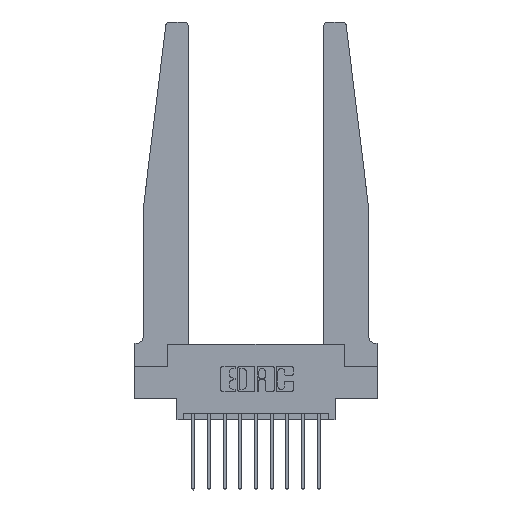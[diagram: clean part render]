
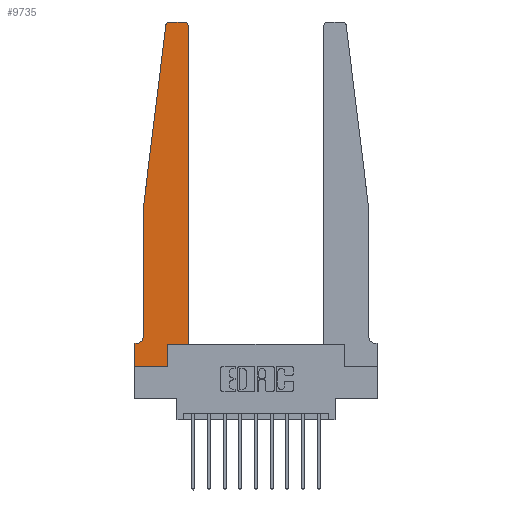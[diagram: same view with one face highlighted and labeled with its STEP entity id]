
A CAD part, top view. The second image highlights one B-rep face of the part: STEP entity #9735.
In plain terms, the highlighted planar face has unit normal (0, 0, 1).
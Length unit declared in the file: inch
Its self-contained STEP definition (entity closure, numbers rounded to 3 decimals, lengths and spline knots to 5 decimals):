
#24 = CARTESIAN_POINT ( 'NONE',  ( 0.27653, 2.72, 0.37 ) ) ;
#117 = VECTOR ( 'NONE', #2844, 39.37008 ) ;
#238 = VERTEX_POINT ( 'NONE', #4999 ) ;
#250 = VERTEX_POINT ( 'NONE', #1416 ) ;
#316 = LINE ( 'NONE', #969, #6239 ) ;
#325 = DIRECTION ( 'NONE',  ( -1., 0., 0. ) ) ;
#347 = LINE ( 'NONE', #9294, #12099 ) ;
#415 = ORIENTED_EDGE ( 'NONE', *, *, #4697, .T. ) ;
#616 = EDGE_CURVE ( 'NONE', #13583, #8417, #14732, .T. ) ;
#830 = CARTESIAN_POINT ( 'NONE',  ( 0.395, 2.72, 0.37 ) ) ;
#891 = ORIENTED_EDGE ( 'NONE', *, *, #8493, .T. ) ;
#969 = CARTESIAN_POINT ( 'NONE',  ( 0.065, 1.25, 0.37 ) ) ;
#978 = EDGE_CURVE ( 'NONE', #8793, #11967, #13027, .T. ) ;
#1045 = CARTESIAN_POINT ( 'NONE',  ( 0.2605, 0.18, 0.37 ) ) ;
#1146 = EDGE_CURVE ( 'NONE', #4837, #238, #4640, .T. ) ;
#1221 = DIRECTION ( 'NONE',  ( 1., 0., 0. ) ) ;
#1333 = ORIENTED_EDGE ( 'NONE', *, *, #1146, .T. ) ;
#1416 = CARTESIAN_POINT ( 'NONE',  ( 0.015, 0.1875, 0.37 ) ) ;
#1560 = EDGE_LOOP ( 'NONE', ( #9236, #891, #6658, #9696, #10769, #415, #2440, #8601, #11842, #1333, #6255, #4592 ) ) ;
#1651 = CARTESIAN_POINT ( 'NONE',  ( 0.065, 1.25, 0.37 ) ) ;
#1719 = CARTESIAN_POINT ( 'NONE',  ( 0.2605, 0.18, 0.37 ) ) ;
#1754 = CARTESIAN_POINT ( 'NONE',  ( 0.425, 0.18, 0.37 ) ) ;
#1831 = EDGE_CURVE ( 'NONE', #12638, #8793, #347, .T. ) ;
#2023 = DIRECTION ( 'NONE',  ( 1., 0., 0. ) ) ;
#2075 = FACE_OUTER_BOUND ( 'NONE', #1560, .T. ) ;
#2248 = DIRECTION ( 'NONE',  ( 0., 1., 0. ) ) ;
#2430 = EDGE_CURVE ( 'NONE', #8417, #10981, #4631, .T. ) ;
#2440 = ORIENTED_EDGE ( 'NONE', *, *, #1831, .T. ) ;
#2844 = DIRECTION ( 'NONE',  ( 0., -1., 0. ) ) ;
#3361 = DIRECTION ( 'NONE',  ( -0.122, -0.992, 0. ) ) ;
#3712 = AXIS2_PLACEMENT_3D ( 'NONE', #14414, #7411, #325 ) ;
#4321 = AXIS2_PLACEMENT_3D ( 'NONE', #830, #9087, #2023 ) ;
#4592 = ORIENTED_EDGE ( 'NONE', *, *, #616, .T. ) ;
#4631 = LINE ( 'NONE', #5752, #10487 ) ;
#4640 = LINE ( 'NONE', #1754, #10501 ) ;
#4697 = EDGE_CURVE ( 'NONE', #250, #12638, #8228, .T. ) ;
#4837 = VERTEX_POINT ( 'NONE', #1719 ) ;
#4999 = CARTESIAN_POINT ( 'NONE',  ( 0.425, 0.18, 0.37 ) ) ;
#5190 = DIRECTION ( 'NONE',  ( 0., 0., 1. ) ) ;
#5752 = CARTESIAN_POINT ( 'NONE',  ( 0.25, 2.75, 0.37 ) ) ;
#6239 = VECTOR ( 'NONE', #3361, 39.37008 ) ;
#6249 = CARTESIAN_POINT ( 'NONE',  ( 0., 0., 0.37 ) ) ;
#6255 = ORIENTED_EDGE ( 'NONE', *, *, #8692, .T. ) ;
#6658 = ORIENTED_EDGE ( 'NONE', *, *, #12564, .T. ) ;
#7308 = CARTESIAN_POINT ( 'NONE',  ( 0.24675, 2.72367, 0.37 ) ) ;
#7411 = DIRECTION ( 'NONE',  ( 0., 0., -1. ) ) ;
#7706 = CARTESIAN_POINT ( 'NONE',  ( 0.425, 2.72, 0.37 ) ) ;
#7771 = CARTESIAN_POINT ( 'NONE',  ( 0.065, 1.25, 0.37 ) ) ;
#8195 = CARTESIAN_POINT ( 'NONE',  ( 0., 0.1875, 0.37 ) ) ;
#8228 = LINE ( 'NONE', #13088, #10969 ) ;
#8288 = DIRECTION ( 'NONE',  ( 0., 0., 1. ) ) ;
#8417 = VERTEX_POINT ( 'NONE', #12748 ) ;
#8493 = EDGE_CURVE ( 'NONE', #10981, #13328, #11287, .T. ) ;
#8601 = ORIENTED_EDGE ( 'NONE', *, *, #978, .T. ) ;
#8645 = CARTESIAN_POINT ( 'NONE',  ( 0.425, 0.18, 0.37 ) ) ;
#8692 = EDGE_CURVE ( 'NONE', #238, #13583, #14959, .T. ) ;
#8731 = CIRCLE ( 'NONE', #3712, 0.05 ) ;
#8793 = VERTEX_POINT ( 'NONE', #14630 ) ;
#9006 = VECTOR ( 'NONE', #2248, 39.37008 ) ;
#9087 = DIRECTION ( 'NONE',  ( 0., 0., 1. ) ) ;
#9177 = EDGE_CURVE ( 'NONE', #10289, #250, #8731, .T. ) ;
#9236 = ORIENTED_EDGE ( 'NONE', *, *, #2430, .T. ) ;
#9294 = CARTESIAN_POINT ( 'NONE',  ( 0., 0., 0.37 ) ) ;
#9696 = ORIENTED_EDGE ( 'NONE', *, *, #12857, .T. ) ;
#9735 = ADVANCED_FACE ( 'NONE', ( #2075 ), #12166, .T. ) ;
#9979 = VECTOR ( 'NONE', #10912, 39.37008 ) ;
#10289 = VERTEX_POINT ( 'NONE', #14479 ) ;
#10487 = VECTOR ( 'NONE', #15109, 39.37008 ) ;
#10501 = VECTOR ( 'NONE', #14646, 39.37008 ) ;
#10769 = ORIENTED_EDGE ( 'NONE', *, *, #9177, .T. ) ;
#10820 = DIRECTION ( 'NONE',  ( -1., 0., 0. ) ) ;
#10912 = DIRECTION ( 'NONE',  ( 1., 0., 0. ) ) ;
#10969 = VECTOR ( 'NONE', #10820, 39.37008 ) ;
#10981 = VERTEX_POINT ( 'NONE', #14509 ) ;
#11155 = LINE ( 'NONE', #1651, #117 ) ;
#11160 = CARTESIAN_POINT ( 'NONE',  ( 0.2605, 0., 0.37 ) ) ;
#11287 = CIRCLE ( 'NONE', #13985, 0.03 ) ;
#11714 = LINE ( 'NONE', #1045, #9006 ) ;
#11813 = VECTOR ( 'NONE', #13322, 39.37008 ) ;
#11842 = ORIENTED_EDGE ( 'NONE', *, *, #12082, .T. ) ;
#11967 = VERTEX_POINT ( 'NONE', #11160 ) ;
#12082 = EDGE_CURVE ( 'NONE', #11967, #4837, #11714, .T. ) ;
#12099 = VECTOR ( 'NONE', #12785, 39.37008 ) ;
#12166 = PLANE ( 'NONE',  #15194 ) ;
#12564 = EDGE_CURVE ( 'NONE', #13328, #12986, #316, .T. ) ;
#12638 = VERTEX_POINT ( 'NONE', #8195 ) ;
#12748 = CARTESIAN_POINT ( 'NONE',  ( 0.395, 2.75, 0.37 ) ) ;
#12785 = DIRECTION ( 'NONE',  ( 0., -1., 0. ) ) ;
#12857 = EDGE_CURVE ( 'NONE', #12986, #10289, #11155, .T. ) ;
#12986 = VERTEX_POINT ( 'NONE', #7771 ) ;
#13027 = LINE ( 'NONE', #6249, #9979 ) ;
#13088 = CARTESIAN_POINT ( 'NONE',  ( 0.065, 0.1875, 0.37 ) ) ;
#13322 = DIRECTION ( 'NONE',  ( 0., 1., 0. ) ) ;
#13328 = VERTEX_POINT ( 'NONE', #7308 ) ;
#13345 = DIRECTION ( 'NONE',  ( 1., 0., 0. ) ) ;
#13583 = VERTEX_POINT ( 'NONE', #7706 ) ;
#13985 = AXIS2_PLACEMENT_3D ( 'NONE', #24, #8288, #1221 ) ;
#14414 = CARTESIAN_POINT ( 'NONE',  ( 0.015, 0.2375, 0.37 ) ) ;
#14479 = CARTESIAN_POINT ( 'NONE',  ( 0.065, 0.2375, 0.37 ) ) ;
#14494 = CARTESIAN_POINT ( 'NONE',  ( 0., 0.1875, 0.37 ) ) ;
#14509 = CARTESIAN_POINT ( 'NONE',  ( 0.27653, 2.75, 0.37 ) ) ;
#14630 = CARTESIAN_POINT ( 'NONE',  ( 0., 0., 0.37 ) ) ;
#14646 = DIRECTION ( 'NONE',  ( 1., 0., 0. ) ) ;
#14732 = CIRCLE ( 'NONE', #4321, 0.03 ) ;
#14959 = LINE ( 'NONE', #8645, #11813 ) ;
#15109 = DIRECTION ( 'NONE',  ( -1., 0., 0. ) ) ;
#15194 = AXIS2_PLACEMENT_3D ( 'NONE', #14494, #5190, #13345 ) ;
